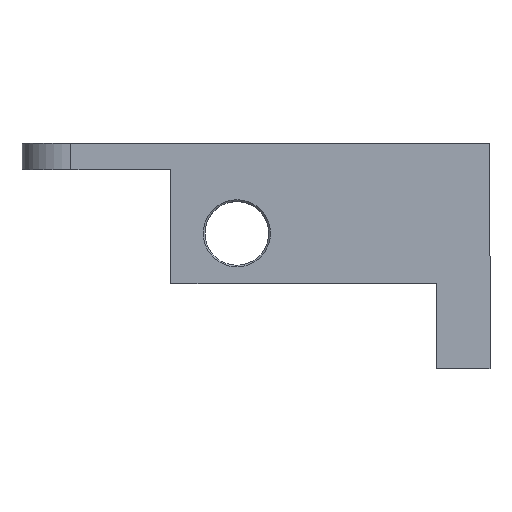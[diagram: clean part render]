
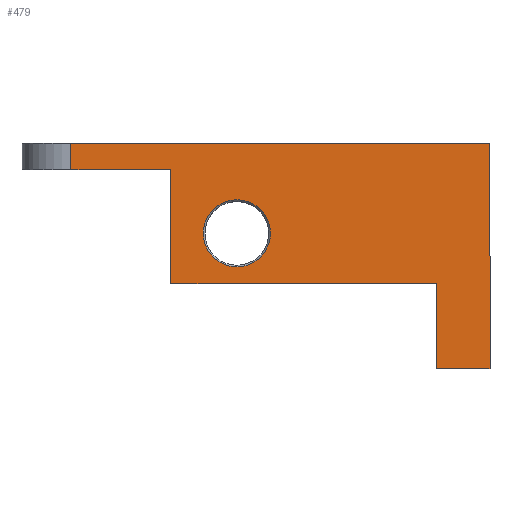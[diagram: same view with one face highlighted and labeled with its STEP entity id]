
A CAD part, top view. The second image highlights one B-rep face of the part: STEP entity #479.
In plain terms, the highlighted planar face has unit normal (0, 0, 1).
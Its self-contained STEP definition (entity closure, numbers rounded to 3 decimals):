
#3 = EDGE_LOOP ( 'NONE', ( #193, #135, #163, #389, #197, #71, #130, #138 ) ) ;
#13 = DIRECTION ( 'NONE',  ( -1., 0., 0. ) ) ;
#14 = DIRECTION ( 'NONE',  ( -1., 0., 0. ) ) ;
#17 = DIRECTION ( 'NONE',  ( 0., 1., 0. ) ) ;
#22 = EDGE_CURVE ( 'NONE', #525, #67, #438, .T. ) ;
#23 = CARTESIAN_POINT ( 'NONE',  ( 0., 0., 1.46 ) ) ;
#24 = CARTESIAN_POINT ( 'NONE',  ( -9.525, -0.794, 1.46 ) ) ;
#27 = DIRECTION ( 'NONE',  ( 0., 0., -1. ) ) ;
#28 = DIRECTION ( 'NONE',  ( 0., 1., 0. ) ) ;
#29 = CARTESIAN_POINT ( 'NONE',  ( -1.588, -6.731, 1.46 ) ) ;
#31 = DIRECTION ( 'NONE',  ( -1., 0., 0. ) ) ;
#35 = CARTESIAN_POINT ( 'NONE',  ( -12.51, -0.794, 1.46 ) ) ;
#37 = AXIS2_PLACEMENT_3D ( 'NONE', #173, #177, #31 ) ;
#54 = DIRECTION ( 'NONE',  ( 0., 0., -1. ) ) ;
#56 = PLANE ( 'NONE',  #414 ) ;
#67 = VERTEX_POINT ( 'NONE', #72 ) ;
#68 = CARTESIAN_POINT ( 'NONE',  ( -6.553, -2.692, 1.46 ) ) ;
#71 = ORIENTED_EDGE ( 'NONE', *, *, #507, .T. ) ;
#72 = CARTESIAN_POINT ( 'NONE',  ( 0., -6.731, 1.46 ) ) ;
#105 = CIRCLE ( 'NONE', #374, 1.003 ) ;
#109 = DIRECTION ( 'NONE',  ( -1., 0., 0. ) ) ;
#112 = CARTESIAN_POINT ( 'NONE',  ( -1.587, -4.191, 1.46 ) ) ;
#118 = CARTESIAN_POINT ( 'NONE',  ( -7.556, -2.692, 1.46 ) ) ;
#128 = DIRECTION ( 'NONE',  ( -1., 0., 0. ) ) ;
#130 = ORIENTED_EDGE ( 'NONE', *, *, #206, .F. ) ;
#135 = ORIENTED_EDGE ( 'NONE', *, *, #399, .F. ) ;
#138 = ORIENTED_EDGE ( 'NONE', *, *, #183, .F. ) ;
#141 = CARTESIAN_POINT ( 'NONE',  ( 0., -6.731, 1.46 ) ) ;
#147 = CARTESIAN_POINT ( 'NONE',  ( -13.97, -0.794, 1.46 ) ) ;
#163 = ORIENTED_EDGE ( 'NONE', *, *, #22, .T. ) ;
#167 = CARTESIAN_POINT ( 'NONE',  ( 0., -6.731, 1.46 ) ) ;
#170 = EDGE_CURVE ( 'NONE', #416, #403, #364, .T. ) ;
#171 = CARTESIAN_POINT ( 'NONE',  ( -9.525, -4.191, 1.46 ) ) ;
#173 = CARTESIAN_POINT ( 'NONE',  ( -7.556, -2.692, 1.46 ) ) ;
#177 = DIRECTION ( 'NONE',  ( 0., 0., -1. ) ) ;
#182 = DIRECTION ( 'NONE',  ( 1., 0., 0. ) ) ;
#183 = EDGE_CURVE ( 'NONE', #397, #252, #444, .T. ) ;
#193 = ORIENTED_EDGE ( 'NONE', *, *, #358, .F. ) ;
#197 = ORIENTED_EDGE ( 'NONE', *, *, #218, .T. ) ;
#206 = EDGE_CURVE ( 'NONE', #252, #377, #515, .T. ) ;
#218 = EDGE_CURVE ( 'NONE', #503, #496, #312, .T. ) ;
#234 = CARTESIAN_POINT ( 'NONE',  ( -1.587, -4.191, 1.46 ) ) ;
#235 = CARTESIAN_POINT ( 'NONE',  ( -12.51, 0., 1.46 ) ) ;
#243 = DIRECTION ( 'NONE',  ( -1., 0., 0. ) ) ;
#244 = CARTESIAN_POINT ( 'NONE',  ( -8.56, -2.692, 1.46 ) ) ;
#249 = CARTESIAN_POINT ( 'NONE',  ( -9.525, -0.794, 1.46 ) ) ;
#252 = VERTEX_POINT ( 'NONE', #24 ) ;
#285 = ORIENTED_EDGE ( 'NONE', *, *, #170, .T. ) ;
#287 = CARTESIAN_POINT ( 'NONE',  ( 0., 0., 1.46 ) ) ;
#304 = VECTOR ( 'NONE', #13, 1000. ) ;
#305 = CARTESIAN_POINT ( 'NONE',  ( -12.51, -6.731, 1.46 ) ) ;
#308 = CARTESIAN_POINT ( 'NONE',  ( 0., 0., 1.46 ) ) ;
#309 = DIRECTION ( 'NONE',  ( 0., -1., 0. ) ) ;
#312 = LINE ( 'NONE', #23, #304 ) ;
#318 = CARTESIAN_POINT ( 'NONE',  ( -1.588, -6.731, 1.46 ) ) ;
#319 = DIRECTION ( 'NONE',  ( 0., 1., 0. ) ) ;
#335 = VECTOR ( 'NONE', #28, 1000. ) ;
#347 = LINE ( 'NONE', #112, #356 ) ;
#356 = VECTOR ( 'NONE', #109, 1000. ) ;
#358 = EDGE_CURVE ( 'NONE', #390, #397, #347, .T. ) ;
#360 = LINE ( 'NONE', #29, #335 ) ;
#364 = CIRCLE ( 'NONE', #37, 1.003 ) ;
#374 = AXIS2_PLACEMENT_3D ( 'NONE', #118, #27, #243 ) ;
#377 = VERTEX_POINT ( 'NONE', #35 ) ;
#388 = FACE_BOUND ( 'NONE', #400, .T. ) ;
#389 = ORIENTED_EDGE ( 'NONE', *, *, #521, .T. ) ;
#390 = VERTEX_POINT ( 'NONE', #234 ) ;
#395 = ORIENTED_EDGE ( 'NONE', *, *, #429, .T. ) ;
#397 = VERTEX_POINT ( 'NONE', #171 ) ;
#399 = EDGE_CURVE ( 'NONE', #525, #390, #360, .T. ) ;
#400 = EDGE_LOOP ( 'NONE', ( #285, #395 ) ) ;
#403 = VERTEX_POINT ( 'NONE', #244 ) ;
#414 = AXIS2_PLACEMENT_3D ( 'NONE', #141, #54, #128 ) ;
#416 = VERTEX_POINT ( 'NONE', #68 ) ;
#429 = EDGE_CURVE ( 'NONE', #403, #416, #105, .T. ) ;
#438 = LINE ( 'NONE', #167, #439 ) ;
#439 = VECTOR ( 'NONE', #182, 1000. ) ;
#444 = LINE ( 'NONE', #249, #456 ) ;
#453 = VECTOR ( 'NONE', #309, 1000. ) ;
#456 = VECTOR ( 'NONE', #17, 1000. ) ;
#460 = LINE ( 'NONE', #305, #453 ) ;
#464 = FACE_OUTER_BOUND ( 'NONE', #3, .T. ) ;
#479 = ADVANCED_FACE ( 'NONE', ( #388, #464 ), #56, .F. ) ;
#492 = LINE ( 'NONE', #308, #519 ) ;
#496 = VERTEX_POINT ( 'NONE', #235 ) ;
#497 = VECTOR ( 'NONE', #14, 1000. ) ;
#503 = VERTEX_POINT ( 'NONE', #287 ) ;
#507 = EDGE_CURVE ( 'NONE', #496, #377, #460, .T. ) ;
#515 = LINE ( 'NONE', #147, #497 ) ;
#519 = VECTOR ( 'NONE', #319, 1000. ) ;
#521 = EDGE_CURVE ( 'NONE', #67, #503, #492, .T. ) ;
#525 = VERTEX_POINT ( 'NONE', #318 ) ;
